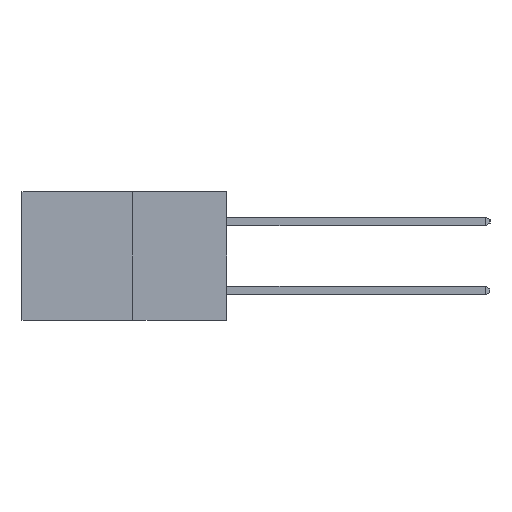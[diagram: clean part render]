
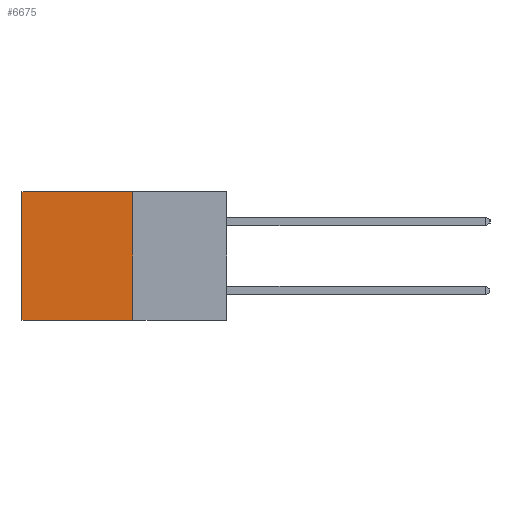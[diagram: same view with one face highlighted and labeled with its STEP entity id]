
A CAD part, left-side view. The second image highlights one B-rep face of the part: STEP entity #6675.
In plain terms, the highlighted planar face has unit normal (-1, 0, 0).
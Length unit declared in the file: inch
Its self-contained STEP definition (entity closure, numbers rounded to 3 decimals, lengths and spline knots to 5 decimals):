
#513 = DIRECTION ( 'NONE',  ( 0., 0., -1. ) ) ;
#610 = VECTOR ( 'NONE', #513, 39.37008 ) ;
#885 = CARTESIAN_POINT ( 'NONE',  ( 0.277, 0.59, 0. ) ) ;
#926 = CARTESIAN_POINT ( 'NONE',  ( 0.277, 0.27, 0. ) ) ;
#1410 = VERTEX_POINT ( 'NONE', #11073 ) ;
#1490 = PLANE ( 'NONE',  #2227 ) ;
#2227 = AXIS2_PLACEMENT_3D ( 'NONE', #8935, #3330, #9853 ) ;
#2552 = ORIENTED_EDGE ( 'NONE', *, *, #4361, .F. ) ;
#2596 = ORIENTED_EDGE ( 'NONE', *, *, #8672, .T. ) ;
#2905 = EDGE_CURVE ( 'NONE', #4500, #8277, #7660, .T. ) ;
#3033 = EDGE_CURVE ( 'NONE', #4500, #9033, #8961, .T. ) ;
#3074 = LINE ( 'NONE', #7046, #610 ) ;
#3330 = DIRECTION ( 'NONE',  ( 1., 0., 0. ) ) ;
#3676 = VECTOR ( 'NONE', #4258, 39.37008 ) ;
#4258 = DIRECTION ( 'NONE',  ( 0., 0., -1. ) ) ;
#4361 = EDGE_CURVE ( 'NONE', #9033, #1410, #9504, .T. ) ;
#4500 = VERTEX_POINT ( 'NONE', #8021 ) ;
#5161 = VECTOR ( 'NONE', #9184, 39.37008 ) ;
#5759 = CARTESIAN_POINT ( 'NONE',  ( 0.277, 0.27, -0.37 ) ) ;
#6675 = ADVANCED_FACE ( 'NONE', ( #9662 ), #1490, .F. ) ;
#7014 = DIRECTION ( 'NONE',  ( 0., 1., 0. ) ) ;
#7046 = CARTESIAN_POINT ( 'NONE',  ( 0.277, 0.59, -0.37 ) ) ;
#7660 = LINE ( 'NONE', #926, #10112 ) ;
#8021 = CARTESIAN_POINT ( 'NONE',  ( 0.277, 0.27, 0. ) ) ;
#8138 = CARTESIAN_POINT ( 'NONE',  ( 0.277, 0.27, -0.37 ) ) ;
#8277 = VERTEX_POINT ( 'NONE', #885 ) ;
#8328 = ORIENTED_EDGE ( 'NONE', *, *, #3033, .F. ) ;
#8672 = EDGE_CURVE ( 'NONE', #8277, #1410, #3074, .T. ) ;
#8935 = CARTESIAN_POINT ( 'NONE',  ( 0.277, 0.27, -0.37 ) ) ;
#8961 = LINE ( 'NONE', #8138, #3676 ) ;
#8983 = EDGE_LOOP ( 'NONE', ( #2596, #2552, #8328, #9439 ) ) ;
#9033 = VERTEX_POINT ( 'NONE', #5759 ) ;
#9184 = DIRECTION ( 'NONE',  ( 0., 1., 0. ) ) ;
#9225 = CARTESIAN_POINT ( 'NONE',  ( 0.277, 0.27, -0.37 ) ) ;
#9439 = ORIENTED_EDGE ( 'NONE', *, *, #2905, .T. ) ;
#9504 = LINE ( 'NONE', #9225, #5161 ) ;
#9662 = FACE_OUTER_BOUND ( 'NONE', #8983, .T. ) ;
#9853 = DIRECTION ( 'NONE',  ( 0., 0., -1. ) ) ;
#10112 = VECTOR ( 'NONE', #7014, 39.37008 ) ;
#11073 = CARTESIAN_POINT ( 'NONE',  ( 0.277, 0.59, -0.37 ) ) ;
